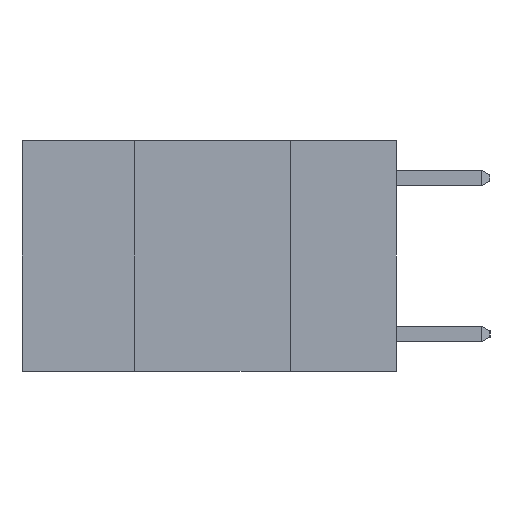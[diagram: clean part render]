
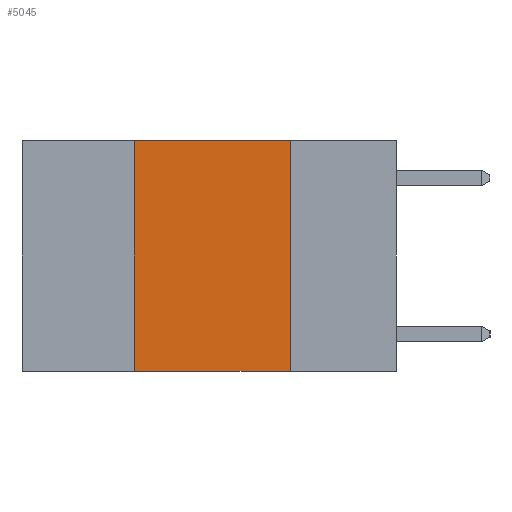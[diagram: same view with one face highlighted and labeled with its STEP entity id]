
A CAD part, left-side view. The second image highlights one B-rep face of the part: STEP entity #5045.
In plain terms, the highlighted planar face has unit normal (-1, 0, 0).
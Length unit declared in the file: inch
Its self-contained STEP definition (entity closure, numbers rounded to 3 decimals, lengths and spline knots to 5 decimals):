
#174 = CARTESIAN_POINT ( 'NONE',  ( 0., 0.17, -0.37 ) ) ;
#790 = EDGE_CURVE ( 'NONE', #8117, #5602, #10597, .T. ) ;
#966 = VERTEX_POINT ( 'NONE', #6501 ) ;
#1033 = AXIS2_PLACEMENT_3D ( 'NONE', #4225, #4257, #10033 ) ;
#1274 = DIRECTION ( 'NONE',  ( 0., 0., -1. ) ) ;
#1617 = EDGE_CURVE ( 'NONE', #966, #8117, #5436, .T. ) ;
#1759 = VECTOR ( 'NONE', #3852, 39.37008 ) ;
#1819 = VECTOR ( 'NONE', #6910, 39.37008 ) ;
#3711 = VERTEX_POINT ( 'NONE', #174 ) ;
#3852 = DIRECTION ( 'NONE',  ( 0., -1., 0. ) ) ;
#3872 = EDGE_CURVE ( 'NONE', #5602, #3711, #4739, .T. ) ;
#4065 = LINE ( 'NONE', #10153, #1819 ) ;
#4225 = CARTESIAN_POINT ( 'NONE',  ( 0., 0.6, 0. ) ) ;
#4257 = DIRECTION ( 'NONE',  ( 1., 0., 0. ) ) ;
#4280 = CARTESIAN_POINT ( 'NONE',  ( 0., 0.17, 0. ) ) ;
#4476 = VECTOR ( 'NONE', #1274, 39.37008 ) ;
#4739 = LINE ( 'NONE', #6274, #4476 ) ;
#4807 = CARTESIAN_POINT ( 'NONE',  ( 0., 0.42, 0. ) ) ;
#5045 = ADVANCED_FACE ( 'NONE', ( #8867 ), #7600, .F. ) ;
#5436 = LINE ( 'NONE', #9435, #8833 ) ;
#5578 = CARTESIAN_POINT ( 'NONE',  ( 0., 0.6, 0. ) ) ;
#5602 = VERTEX_POINT ( 'NONE', #4280 ) ;
#5754 = DIRECTION ( 'NONE',  ( 0., 0., 1. ) ) ;
#6274 = CARTESIAN_POINT ( 'NONE',  ( 0., 0.17, 0. ) ) ;
#6501 = CARTESIAN_POINT ( 'NONE',  ( 0., 0.42, -0.37 ) ) ;
#6694 = ORIENTED_EDGE ( 'NONE', *, *, #8550, .T. ) ;
#6910 = DIRECTION ( 'NONE',  ( 0., -1., 0. ) ) ;
#7079 = ORIENTED_EDGE ( 'NONE', *, *, #1617, .F. ) ;
#7600 = PLANE ( 'NONE',  #1033 ) ;
#7888 = ORIENTED_EDGE ( 'NONE', *, *, #3872, .F. ) ;
#8117 = VERTEX_POINT ( 'NONE', #4807 ) ;
#8251 = ORIENTED_EDGE ( 'NONE', *, *, #790, .F. ) ;
#8550 = EDGE_CURVE ( 'NONE', #966, #3711, #4065, .T. ) ;
#8833 = VECTOR ( 'NONE', #5754, 39.37008 ) ;
#8867 = FACE_OUTER_BOUND ( 'NONE', #9660, .T. ) ;
#9435 = CARTESIAN_POINT ( 'NONE',  ( 0., 0.42, 0. ) ) ;
#9660 = EDGE_LOOP ( 'NONE', ( #7888, #8251, #7079, #6694 ) ) ;
#10033 = DIRECTION ( 'NONE',  ( 0., 0., -1. ) ) ;
#10153 = CARTESIAN_POINT ( 'NONE',  ( 0., 0.6, -0.37 ) ) ;
#10597 = LINE ( 'NONE', #5578, #1759 ) ;
